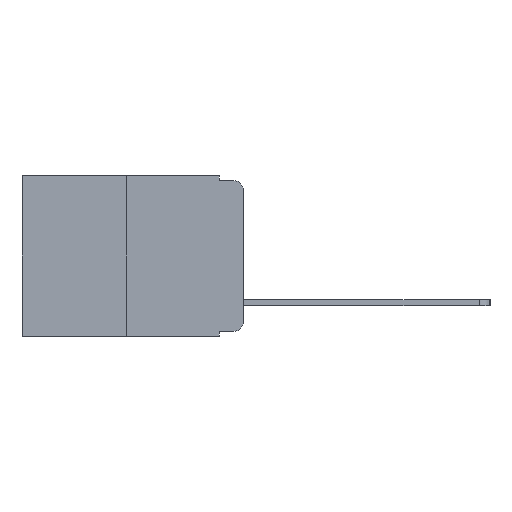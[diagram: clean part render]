
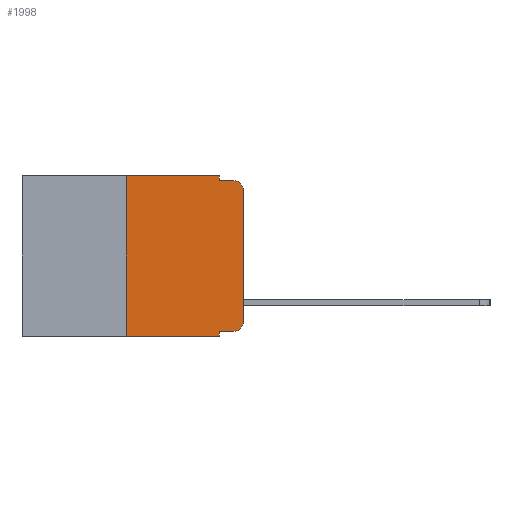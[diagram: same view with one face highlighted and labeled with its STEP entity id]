
A CAD part, left-side view. The second image highlights one B-rep face of the part: STEP entity #1998.
In plain terms, the highlighted planar face has unit normal (-1, 0, 0).
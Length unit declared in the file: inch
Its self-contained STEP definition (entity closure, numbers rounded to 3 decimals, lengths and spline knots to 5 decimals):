
#320 = LINE ( 'NONE', #12434, #15972 ) ;
#844 = ORIENTED_EDGE ( 'NONE', *, *, #12496, .T. ) ;
#1034 = DIRECTION ( 'NONE',  ( 0., -1., 0. ) ) ;
#1106 = LINE ( 'NONE', #7829, #4239 ) ;
#1288 = EDGE_CURVE ( 'NONE', #15786, #12847, #7975, .T. ) ;
#1324 = DIRECTION ( 'NONE',  ( 0., 0., -1. ) ) ;
#1524 = CARTESIAN_POINT ( 'NONE',  ( 0., 0.02, -0.03 ) ) ;
#1570 = CARTESIAN_POINT ( 'NONE',  ( 0., 0., -0.03 ) ) ;
#1603 = VECTOR ( 'NONE', #6996, 39.37008 ) ;
#1998 = ADVANCED_FACE ( 'NONE', ( #5357 ), #13465, .F. ) ;
#2168 = EDGE_CURVE ( 'NONE', #7659, #15786, #5152, .T. ) ;
#2492 = ORIENTED_EDGE ( 'NONE', *, *, #5925, .T. ) ;
#2651 = LINE ( 'NONE', #5908, #9198 ) ;
#2841 = DIRECTION ( 'NONE',  ( 0., 0., -1. ) ) ;
#2919 = ORIENTED_EDGE ( 'NONE', *, *, #2168, .T. ) ;
#2995 = DIRECTION ( 'NONE',  ( 0., -1., 0. ) ) ;
#2998 = CARTESIAN_POINT ( 'NONE',  ( 0., 0., 0. ) ) ;
#3957 = EDGE_CURVE ( 'NONE', #7659, #14490, #2651, .T. ) ;
#4239 = VECTOR ( 'NONE', #1324, 39.37008 ) ;
#4487 = VECTOR ( 'NONE', #2995, 39.37008 ) ;
#4601 = VECTOR ( 'NONE', #1034, 39.37008 ) ;
#4780 = CIRCLE ( 'NONE', #13183, 0.02 ) ;
#4822 = ORIENTED_EDGE ( 'NONE', *, *, #8325, .F. ) ;
#4837 = DIRECTION ( 'NONE',  ( 1., 0., 0. ) ) ;
#4874 = EDGE_CURVE ( 'NONE', #14850, #9640, #320, .T. ) ;
#4921 = CARTESIAN_POINT ( 'NONE',  ( 0., 0.473, 0. ) ) ;
#5052 = DIRECTION ( 'NONE',  ( 0., 0., -1. ) ) ;
#5068 = CARTESIAN_POINT ( 'NONE',  ( 0., 0.051, -0.01 ) ) ;
#5152 = LINE ( 'NONE', #15170, #1603 ) ;
#5357 = FACE_OUTER_BOUND ( 'NONE', #7076, .T. ) ;
#5404 = CARTESIAN_POINT ( 'NONE',  ( 0., 0.25, 0. ) ) ;
#5908 = CARTESIAN_POINT ( 'NONE',  ( 0., 0.051, 0. ) ) ;
#5925 = EDGE_CURVE ( 'NONE', #14850, #14490, #7930, .T. ) ;
#6057 = ORIENTED_EDGE ( 'NONE', *, *, #3957, .F. ) ;
#6629 = EDGE_CURVE ( 'NONE', #7408, #12029, #1106, .T. ) ;
#6996 = DIRECTION ( 'NONE',  ( 0., -1., 0. ) ) ;
#7076 = EDGE_LOOP ( 'NONE', ( #844, #7850, #4822, #8240, #11974, #12345, #2492, #6057, #2919, #13076 ) ) ;
#7112 = CARTESIAN_POINT ( 'NONE',  ( 0., 0.473, 0. ) ) ;
#7408 = VERTEX_POINT ( 'NONE', #12092 ) ;
#7659 = VERTEX_POINT ( 'NONE', #11318 ) ;
#7829 = CARTESIAN_POINT ( 'NONE',  ( 0., 0.051, 0. ) ) ;
#7849 = VECTOR ( 'NONE', #13679, 39.37008 ) ;
#7850 = ORIENTED_EDGE ( 'NONE', *, *, #10925, .T. ) ;
#7859 = DIRECTION ( 'NONE',  ( 0., 0., 1. ) ) ;
#7930 = LINE ( 'NONE', #14607, #4487 ) ;
#7975 = CIRCLE ( 'NONE', #8983, 0.02 ) ;
#8240 = ORIENTED_EDGE ( 'NONE', *, *, #6629, .F. ) ;
#8325 = EDGE_CURVE ( 'NONE', #12029, #11423, #14561, .T. ) ;
#8573 = DIRECTION ( 'NONE',  ( 0., 0., -1. ) ) ;
#8578 = VERTEX_POINT ( 'NONE', #1570 ) ;
#8942 = VECTOR ( 'NONE', #10804, 39.37008 ) ;
#8983 = AXIS2_PLACEMENT_3D ( 'NONE', #15994, #14132, #14182 ) ;
#9198 = VECTOR ( 'NONE', #8573, 39.37008 ) ;
#9640 = VERTEX_POINT ( 'NONE', #5404 ) ;
#9880 = CARTESIAN_POINT ( 'NONE',  ( 0., 0.02, -0.333 ) ) ;
#10661 = DIRECTION ( 'NONE',  ( -1., 0., 0. ) ) ;
#10804 = DIRECTION ( 'NONE',  ( 0., 0., 1. ) ) ;
#10925 = EDGE_CURVE ( 'NONE', #8578, #11423, #4780, .T. ) ;
#11318 = CARTESIAN_POINT ( 'NONE',  ( 0., 0.051, -0.333 ) ) ;
#11423 = VERTEX_POINT ( 'NONE', #16354 ) ;
#11741 = AXIS2_PLACEMENT_3D ( 'NONE', #7112, #4837, #5052 ) ;
#11974 = ORIENTED_EDGE ( 'NONE', *, *, #15263, .F. ) ;
#12029 = VERTEX_POINT ( 'NONE', #13455 ) ;
#12092 = CARTESIAN_POINT ( 'NONE',  ( 0., 0.051, 0. ) ) ;
#12251 = LINE ( 'NONE', #2998, #8942 ) ;
#12345 = ORIENTED_EDGE ( 'NONE', *, *, #4874, .F. ) ;
#12434 = CARTESIAN_POINT ( 'NONE',  ( 0., 0.25, 0. ) ) ;
#12496 = EDGE_CURVE ( 'NONE', #12847, #8578, #12251, .T. ) ;
#12847 = VERTEX_POINT ( 'NONE', #13928 ) ;
#13076 = ORIENTED_EDGE ( 'NONE', *, *, #1288, .T. ) ;
#13183 = AXIS2_PLACEMENT_3D ( 'NONE', #1524, #10661, #2841 ) ;
#13455 = CARTESIAN_POINT ( 'NONE',  ( 0., 0.051, -0.01 ) ) ;
#13465 = PLANE ( 'NONE',  #11741 ) ;
#13475 = LINE ( 'NONE', #4921, #7849 ) ;
#13679 = DIRECTION ( 'NONE',  ( 0., -1., 0. ) ) ;
#13735 = CARTESIAN_POINT ( 'NONE',  ( 0., 0.25, -0.343 ) ) ;
#13928 = CARTESIAN_POINT ( 'NONE',  ( 0., 0., -0.313 ) ) ;
#14132 = DIRECTION ( 'NONE',  ( -1., 0., 0. ) ) ;
#14182 = DIRECTION ( 'NONE',  ( 0., 0., -1. ) ) ;
#14490 = VERTEX_POINT ( 'NONE', #15408 ) ;
#14561 = LINE ( 'NONE', #5068, #4601 ) ;
#14607 = CARTESIAN_POINT ( 'NONE',  ( 0., 0.473, -0.343 ) ) ;
#14850 = VERTEX_POINT ( 'NONE', #13735 ) ;
#15170 = CARTESIAN_POINT ( 'NONE',  ( 0., 0.051, -0.333 ) ) ;
#15263 = EDGE_CURVE ( 'NONE', #9640, #7408, #13475, .T. ) ;
#15408 = CARTESIAN_POINT ( 'NONE',  ( 0., 0.051, -0.343 ) ) ;
#15786 = VERTEX_POINT ( 'NONE', #9880 ) ;
#15972 = VECTOR ( 'NONE', #7859, 39.37008 ) ;
#15994 = CARTESIAN_POINT ( 'NONE',  ( 0., 0.02, -0.313 ) ) ;
#16354 = CARTESIAN_POINT ( 'NONE',  ( 0., 0.02, -0.01 ) ) ;
